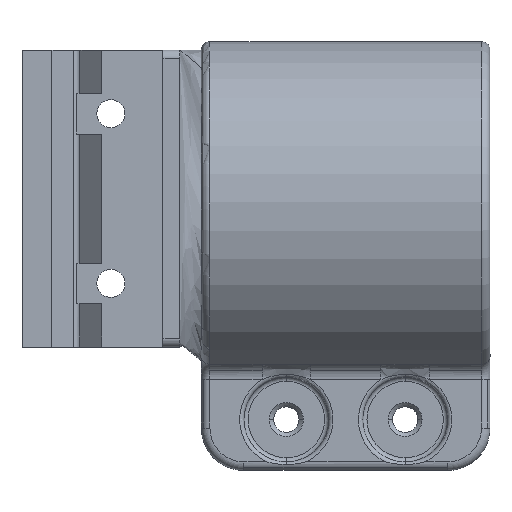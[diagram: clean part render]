
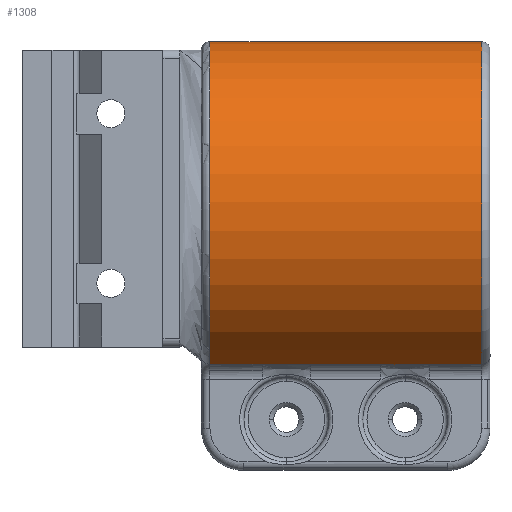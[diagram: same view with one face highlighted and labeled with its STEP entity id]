
A CAD part, front view. The second image highlights one B-rep face of the part: STEP entity #1308.
In plain terms, the highlighted cylindrical face has radius 20 mm (diameter 40 mm), a partial arc.
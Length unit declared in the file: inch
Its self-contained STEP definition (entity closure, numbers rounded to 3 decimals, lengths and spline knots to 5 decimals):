
#134 = VECTOR ( 'NONE', #8714, 39.37008 ) ;
#254 = B_SPLINE_CURVE_WITH_KNOTS ( 'NONE', 3,
 ( #6548, #12241, #11092, #10878, #10034, #538, #14644 ),
 .UNSPECIFIED., .F., .F.,
 ( 4, 1, 1, 1, 4 ),
 ( 0., 0.14286, 0.42857, 0.71429, 1. ),
 .UNSPECIFIED. ) ;
#426 = AXIS2_PLACEMENT_3D ( 'NONE', #789, #14389, #7644 ) ;
#538 = CARTESIAN_POINT ( 'NONE',  ( 1.13485, -1.12742, -1.45824 ) ) ;
#654 = CARTESIAN_POINT ( 'NONE',  ( 0.83228, -1.12742, -1.45824 ) ) ;
#789 = CARTESIAN_POINT ( 'NONE',  ( 0.83228, -0.7874, -0.74803 ) ) ;
#1139 = CARTESIAN_POINT ( 'NONE',  ( 1.33862, -1.12742, -1.45824 ) ) ;
#1308 = ADVANCED_FACE ( 'NONE', ( #9852 ), #1839, .T. ) ;
#1593 = ORIENTED_EDGE ( 'NONE', *, *, #7094, .F. ) ;
#1711 = CARTESIAN_POINT ( 'NONE',  ( 0.87165, -0.7874, 0.03937 ) ) ;
#1839 = CYLINDRICAL_SURFACE ( 'NONE', #426, 0.7874 ) ;
#1858 = VERTEX_POINT ( 'NONE', #1139 ) ;
#2294 = CARTESIAN_POINT ( 'NONE',  ( 1.66453, -1.12742, -1.45824 ) ) ;
#2356 = ORIENTED_EDGE ( 'NONE', *, *, #6729, .F. ) ;
#2392 = VERTEX_POINT ( 'NONE', #6885 ) ;
#2494 = CARTESIAN_POINT ( 'NONE',  ( 1.11335, -1.12742, -1.45824 ) ) ;
#2589 = CARTESIAN_POINT ( 'NONE',  ( 1.72878, -1.12339, -1.46016 ) ) ;
#3172 = LINE ( 'NONE', #10198, #9737 ) ;
#3458 = VERTEX_POINT ( 'NONE', #6354 ) ;
#3575 = CARTESIAN_POINT ( 'NONE',  ( 1.8898, -1.12742, -1.45824 ) ) ;
#3659 = EDGE_CURVE ( 'NONE', #3458, #6417, #14049, .T. ) ;
#3844 = CARTESIAN_POINT ( 'NONE',  ( 1.66453, -1.12742, -1.45824 ) ) ;
#4084 = LINE ( 'NONE', #6420, #13623 ) ;
#4477 = VERTEX_POINT ( 'NONE', #2494 ) ;
#5078 = CARTESIAN_POINT ( 'NONE',  ( 2.1315, -0.7874, -0.74803 ) ) ;
#5915 = CARTESIAN_POINT ( 'NONE',  ( 0.83228, -0.7874, 0.03937 ) ) ;
#5930 = CARTESIAN_POINT ( 'NONE',  ( 1.8898, -1.12742, -1.45824 ) ) ;
#6292 = B_SPLINE_CURVE_WITH_KNOTS ( 'NONE', 3,
 ( #3575, #10378, #8029, #8178, #2589, #12653, #2294 ),
 .UNSPECIFIED., .F., .F.,
 ( 4, 1, 1, 1, 4 ),
 ( 0., 0.28571, 0.42857, 0.71429, 1. ),
 .UNSPECIFIED. ) ;
#6354 = CARTESIAN_POINT ( 'NONE',  ( 0.87165, -1.12742, -1.45824 ) ) ;
#6367 = LINE ( 'NONE', #654, #134 ) ;
#6417 = VERTEX_POINT ( 'NONE', #1711 ) ;
#6420 = CARTESIAN_POINT ( 'NONE',  ( 0.83228, -1.12742, -1.45824 ) ) ;
#6548 = CARTESIAN_POINT ( 'NONE',  ( 1.33862, -1.12742, -1.45824 ) ) ;
#6710 = EDGE_CURVE ( 'NONE', #2392, #12735, #10721, .T. ) ;
#6729 = EDGE_CURVE ( 'NONE', #4477, #3458, #6367, .T. ) ;
#6885 = CARTESIAN_POINT ( 'NONE',  ( 2.1315, -0.7874, 0.03937 ) ) ;
#7094 = EDGE_CURVE ( 'NONE', #8059, #1858, #4084, .T. ) ;
#7268 = DIRECTION ( 'NONE',  ( 0., 0., 1. ) ) ;
#7510 = ORIENTED_EDGE ( 'NONE', *, *, #13950, .F. ) ;
#7644 = DIRECTION ( 'NONE',  ( 0., 0., 1. ) ) ;
#7765 = DIRECTION ( 'NONE',  ( -1., 0., 0. ) ) ;
#8029 = CARTESIAN_POINT ( 'NONE',  ( 1.83619, -1.12468, -1.45954 ) ) ;
#8059 = VERTEX_POINT ( 'NONE', #3844 ) ;
#8156 = EDGE_CURVE ( 'NONE', #1858, #4477, #254, .T. ) ;
#8178 = CARTESIAN_POINT ( 'NONE',  ( 1.78257, -1.12069, -1.46142 ) ) ;
#8246 = AXIS2_PLACEMENT_3D ( 'NONE', #9907, #13536, #11332 ) ;
#8550 = DIRECTION ( 'NONE',  ( -1., 0., 0. ) ) ;
#8567 = ORIENTED_EDGE ( 'NONE', *, *, #6710, .F. ) ;
#8714 = DIRECTION ( 'NONE',  ( -1., 0., 0. ) ) ;
#9694 = EDGE_LOOP ( 'NONE', ( #7510, #9932, #2356, #13425, #1593, #13573, #13136, #8567 ) ) ;
#9698 = DIRECTION ( 'NONE',  ( 1., 0., 0. ) ) ;
#9737 = VECTOR ( 'NONE', #7765, 39.37008 ) ;
#9835 = VERTEX_POINT ( 'NONE', #5930 ) ;
#9852 = FACE_OUTER_BOUND ( 'NONE', #9694, .T. ) ;
#9907 = CARTESIAN_POINT ( 'NONE',  ( 0.87165, -0.7874, -0.74803 ) ) ;
#9932 = ORIENTED_EDGE ( 'NONE', *, *, #3659, .F. ) ;
#10034 = CARTESIAN_POINT ( 'NONE',  ( 1.17757, -1.12333, -1.46018 ) ) ;
#10198 = CARTESIAN_POINT ( 'NONE',  ( 0.83228, -1.12742, -1.45824 ) ) ;
#10378 = CARTESIAN_POINT ( 'NONE',  ( 1.8683, -1.12742, -1.45824 ) ) ;
#10525 = DIRECTION ( 'NONE',  ( 1., 0., 0. ) ) ;
#10721 = CIRCLE ( 'NONE', #11937, 0.7874 ) ;
#10878 = CARTESIAN_POINT ( 'NONE',  ( 1.24215, -1.12021, -1.46164 ) ) ;
#11092 = CARTESIAN_POINT ( 'NONE',  ( 1.29566, -1.1262, -1.45882 ) ) ;
#11200 = EDGE_CURVE ( 'NONE', #9835, #8059, #6292, .T. ) ;
#11332 = DIRECTION ( 'NONE',  ( 0., 0., 1. ) ) ;
#11651 = LINE ( 'NONE', #5915, #11683 ) ;
#11683 = VECTOR ( 'NONE', #10525, 39.37008 ) ;
#11887 = CARTESIAN_POINT ( 'NONE',  ( 2.1315, -1.12742, -1.45824 ) ) ;
#11937 = AXIS2_PLACEMENT_3D ( 'NONE', #5078, #9698, #7268 ) ;
#12241 = CARTESIAN_POINT ( 'NONE',  ( 1.32787, -1.12742, -1.45824 ) ) ;
#12357 = EDGE_CURVE ( 'NONE', #12735, #9835, #3172, .T. ) ;
#12653 = CARTESIAN_POINT ( 'NONE',  ( 1.68604, -1.12742, -1.45824 ) ) ;
#12735 = VERTEX_POINT ( 'NONE', #11887 ) ;
#13136 = ORIENTED_EDGE ( 'NONE', *, *, #12357, .F. ) ;
#13425 = ORIENTED_EDGE ( 'NONE', *, *, #8156, .F. ) ;
#13536 = DIRECTION ( 'NONE',  ( -1., 0., 0. ) ) ;
#13573 = ORIENTED_EDGE ( 'NONE', *, *, #11200, .F. ) ;
#13623 = VECTOR ( 'NONE', #8550, 39.37008 ) ;
#13950 = EDGE_CURVE ( 'NONE', #6417, #2392, #11651, .T. ) ;
#14049 = CIRCLE ( 'NONE', #8246, 0.7874 ) ;
#14389 = DIRECTION ( 'NONE',  ( 1., 0., 0. ) ) ;
#14644 = CARTESIAN_POINT ( 'NONE',  ( 1.11335, -1.12742, -1.45824 ) ) ;
